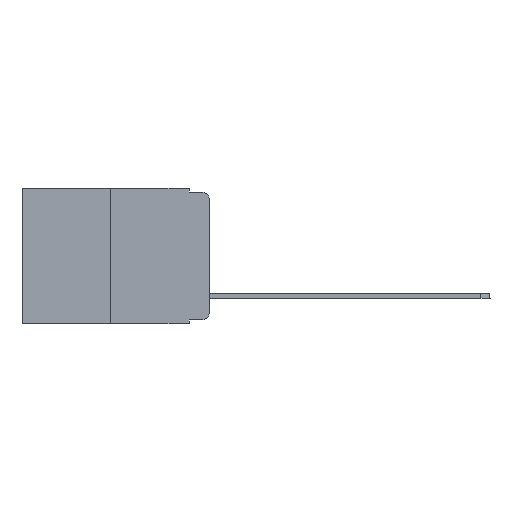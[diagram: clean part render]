
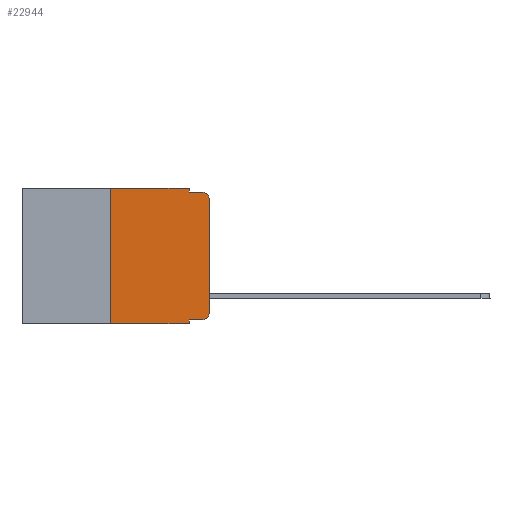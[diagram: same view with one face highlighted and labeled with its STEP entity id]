
A CAD part, left-side view. The second image highlights one B-rep face of the part: STEP entity #22944.
In plain terms, the highlighted planar face has unit normal (-1, 0, 0).
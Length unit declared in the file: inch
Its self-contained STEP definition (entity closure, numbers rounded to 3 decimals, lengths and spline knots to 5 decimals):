
#182 = DIRECTION ( 'NONE',  ( -1., 0., 0. ) ) ;
#783 = VERTEX_POINT ( 'NONE', #9935 ) ;
#1014 = DIRECTION ( 'NONE',  ( 0., 0., 1. ) ) ;
#1089 = CARTESIAN_POINT ( 'NONE',  ( 0., 0.02, -0.03 ) ) ;
#1124 = ORIENTED_EDGE ( 'NONE', *, *, #2728, .T. ) ;
#1665 = LINE ( 'NONE', #3934, #10620 ) ;
#2078 = VECTOR ( 'NONE', #9337, 39.37008 ) ;
#2222 = EDGE_LOOP ( 'NONE', ( #3380, #18162, #15658, #8910, #11755, #12676, #5386, #16366, #9995, #1124 ) ) ;
#2331 = DIRECTION ( 'NONE',  ( 0., 0., -1. ) ) ;
#2564 = VECTOR ( 'NONE', #1014, 39.37008 ) ;
#2728 = EDGE_CURVE ( 'NONE', #783, #10752, #10033, .T. ) ;
#3380 = ORIENTED_EDGE ( 'NONE', *, *, #25067, .T. ) ;
#3476 = CARTESIAN_POINT ( 'NONE',  ( 0., 0.051, -0.01 ) ) ;
#3934 = CARTESIAN_POINT ( 'NONE',  ( 0., 0.473, -0.343 ) ) ;
#4157 = DIRECTION ( 'NONE',  ( 0., 0., -1. ) ) ;
#4929 = CIRCLE ( 'NONE', #9883, 0.02 ) ;
#5085 = CARTESIAN_POINT ( 'NONE',  ( 0., 0., 0. ) ) ;
#5205 = EDGE_CURVE ( 'NONE', #13843, #11909, #7120, .T. ) ;
#5386 = ORIENTED_EDGE ( 'NONE', *, *, #15171, .T. ) ;
#5426 = CARTESIAN_POINT ( 'NONE',  ( 0., 0.25, -0.343 ) ) ;
#5460 = VERTEX_POINT ( 'NONE', #15118 ) ;
#5729 = LINE ( 'NONE', #8693, #23748 ) ;
#5866 = CARTESIAN_POINT ( 'NONE',  ( 0., 0.051, 0. ) ) ;
#6260 = EDGE_CURVE ( 'NONE', #17840, #5460, #19924, .T. ) ;
#6757 = DIRECTION ( 'NONE',  ( 0., 0., -1. ) ) ;
#6995 = VERTEX_POINT ( 'NONE', #16933 ) ;
#7045 = FACE_OUTER_BOUND ( 'NONE', #2222, .T. ) ;
#7120 = LINE ( 'NONE', #19704, #8010 ) ;
#7851 = CARTESIAN_POINT ( 'NONE',  ( 0., 0.02, -0.313 ) ) ;
#8010 = VECTOR ( 'NONE', #19779, 39.37008 ) ;
#8693 = CARTESIAN_POINT ( 'NONE',  ( 0., 0.051, -0.333 ) ) ;
#8910 = ORIENTED_EDGE ( 'NONE', *, *, #20194, .F. ) ;
#9196 = DIRECTION ( 'NONE',  ( 0., 0., -1. ) ) ;
#9337 = DIRECTION ( 'NONE',  ( 0., -1., 0. ) ) ;
#9614 = DIRECTION ( 'NONE',  ( 1., 0., 0. ) ) ;
#9883 = AXIS2_PLACEMENT_3D ( 'NONE', #1089, #18784, #9196 ) ;
#9935 = CARTESIAN_POINT ( 'NONE',  ( 0., 0.02, -0.333 ) ) ;
#9995 = ORIENTED_EDGE ( 'NONE', *, *, #20870, .T. ) ;
#10033 = CIRCLE ( 'NONE', #20353, 0.02 ) ;
#10089 = CARTESIAN_POINT ( 'NONE',  ( 0., 0.051, 0. ) ) ;
#10519 = VERTEX_POINT ( 'NONE', #18118 ) ;
#10620 = VECTOR ( 'NONE', #22334, 39.37008 ) ;
#10752 = VERTEX_POINT ( 'NONE', #14678 ) ;
#10768 = DIRECTION ( 'NONE',  ( 0., -1., 0. ) ) ;
#11755 = ORIENTED_EDGE ( 'NONE', *, *, #12446, .F. ) ;
#11909 = VERTEX_POINT ( 'NONE', #16625 ) ;
#12446 = EDGE_CURVE ( 'NONE', #11909, #16422, #18540, .T. ) ;
#12676 = ORIENTED_EDGE ( 'NONE', *, *, #5205, .F. ) ;
#13221 = VECTOR ( 'NONE', #2331, 39.37008 ) ;
#13592 = PLANE ( 'NONE',  #20812 ) ;
#13843 = VERTEX_POINT ( 'NONE', #5426 ) ;
#13960 = LINE ( 'NONE', #16466, #20417 ) ;
#14334 = CARTESIAN_POINT ( 'NONE',  ( 0., 0.051, -0.333 ) ) ;
#14358 = DIRECTION ( 'NONE',  ( 0., -1., 0. ) ) ;
#14678 = CARTESIAN_POINT ( 'NONE',  ( 0., 0., -0.313 ) ) ;
#15024 = EDGE_CURVE ( 'NONE', #10519, #20297, #4929, .T. ) ;
#15118 = CARTESIAN_POINT ( 'NONE',  ( 0., 0.051, -0.343 ) ) ;
#15171 = EDGE_CURVE ( 'NONE', #13843, #5460, #1665, .T. ) ;
#15658 = ORIENTED_EDGE ( 'NONE', *, *, #18738, .F. ) ;
#16366 = ORIENTED_EDGE ( 'NONE', *, *, #6260, .F. ) ;
#16422 = VERTEX_POINT ( 'NONE', #5866 ) ;
#16466 = CARTESIAN_POINT ( 'NONE',  ( 0., 0.051, 0. ) ) ;
#16625 = CARTESIAN_POINT ( 'NONE',  ( 0., 0.25, 0. ) ) ;
#16812 = LINE ( 'NONE', #3476, #2078 ) ;
#16933 = CARTESIAN_POINT ( 'NONE',  ( 0., 0.051, -0.01 ) ) ;
#17187 = DIRECTION ( 'NONE',  ( 0., 0., -1. ) ) ;
#17298 = LINE ( 'NONE', #5085, #2564 ) ;
#17840 = VERTEX_POINT ( 'NONE', #14334 ) ;
#18118 = CARTESIAN_POINT ( 'NONE',  ( 0., 0., -0.03 ) ) ;
#18162 = ORIENTED_EDGE ( 'NONE', *, *, #15024, .T. ) ;
#18540 = LINE ( 'NONE', #20111, #22831 ) ;
#18738 = EDGE_CURVE ( 'NONE', #6995, #20297, #16812, .T. ) ;
#18784 = DIRECTION ( 'NONE',  ( -1., 0., 0. ) ) ;
#19704 = CARTESIAN_POINT ( 'NONE',  ( 0., 0.25, 0. ) ) ;
#19779 = DIRECTION ( 'NONE',  ( 0., 0., 1. ) ) ;
#19924 = LINE ( 'NONE', #10089, #13221 ) ;
#20111 = CARTESIAN_POINT ( 'NONE',  ( 0., 0.473, 0. ) ) ;
#20194 = EDGE_CURVE ( 'NONE', #16422, #6995, #13960, .T. ) ;
#20297 = VERTEX_POINT ( 'NONE', #22618 ) ;
#20353 = AXIS2_PLACEMENT_3D ( 'NONE', #7851, #182, #4157 ) ;
#20417 = VECTOR ( 'NONE', #6757, 39.37008 ) ;
#20812 = AXIS2_PLACEMENT_3D ( 'NONE', #21444, #9614, #17187 ) ;
#20870 = EDGE_CURVE ( 'NONE', #17840, #783, #5729, .T. ) ;
#21444 = CARTESIAN_POINT ( 'NONE',  ( 0., 0.473, 0. ) ) ;
#22334 = DIRECTION ( 'NONE',  ( 0., -1., 0. ) ) ;
#22618 = CARTESIAN_POINT ( 'NONE',  ( 0., 0.02, -0.01 ) ) ;
#22831 = VECTOR ( 'NONE', #14358, 39.37008 ) ;
#22944 = ADVANCED_FACE ( 'NONE', ( #7045 ), #13592, .F. ) ;
#23748 = VECTOR ( 'NONE', #10768, 39.37008 ) ;
#25067 = EDGE_CURVE ( 'NONE', #10752, #10519, #17298, .T. ) ;
